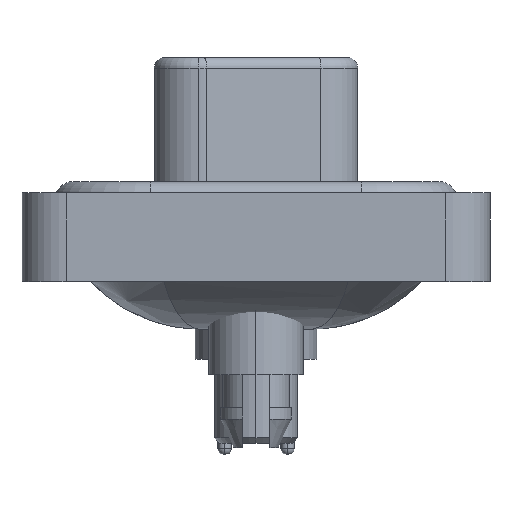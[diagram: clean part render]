
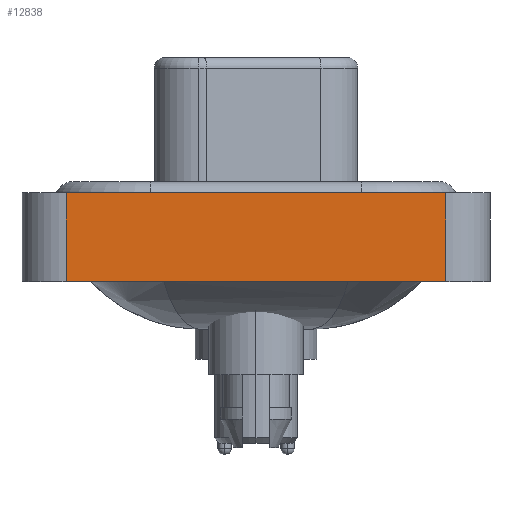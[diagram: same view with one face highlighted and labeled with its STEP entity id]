
A CAD part, left-side view. The second image highlights one B-rep face of the part: STEP entity #12838.
In plain terms, the highlighted planar face has unit normal (-1, 0, 0).
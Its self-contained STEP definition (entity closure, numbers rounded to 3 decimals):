
#242 = DIRECTION ( 'NONE',  ( 0., -1., 0. ) ) ;
#1107 = ORIENTED_EDGE ( 'NONE', *, *, #14644, .F. ) ;
#1788 = FACE_OUTER_BOUND ( 'NONE', #9167, .T. ) ;
#2970 = VERTEX_POINT ( 'NONE', #6866 ) ;
#3926 = VERTEX_POINT ( 'NONE', #19527 ) ;
#4065 = VECTOR ( 'NONE', #242, 1000. ) ;
#4536 = EDGE_CURVE ( 'NONE', #9618, #3926, #15496, .T. ) ;
#5072 = CARTESIAN_POINT ( 'NONE',  ( -7.3, -8.55, -3.6 ) ) ;
#5368 = LINE ( 'NONE', #8829, #6165 ) ;
#6165 = VECTOR ( 'NONE', #19513, 1000. ) ;
#6378 = LINE ( 'NONE', #14205, #4065 ) ;
#6866 = CARTESIAN_POINT ( 'NONE',  ( -7.3, -8.55, 0.4 ) ) ;
#8171 = CARTESIAN_POINT ( 'NONE',  ( -7.3, -8.55, -3.6 ) ) ;
#8829 = CARTESIAN_POINT ( 'NONE',  ( -7.3, -8.55, 0.4 ) ) ;
#9164 = VERTEX_POINT ( 'NONE', #8171 ) ;
#9167 = EDGE_LOOP ( 'NONE', ( #17342, #1107, #18517, #16993 ) ) ;
#9552 = DIRECTION ( 'NONE',  ( 0., 0., 1. ) ) ;
#9618 = VERTEX_POINT ( 'NONE', #12909 ) ;
#11034 = DIRECTION ( 'NONE',  ( -1., 0., 0. ) ) ;
#11043 = VECTOR ( 'NONE', #9552, 1000. ) ;
#12065 = EDGE_CURVE ( 'NONE', #9618, #9164, #6378, .T. ) ;
#12542 = CARTESIAN_POINT ( 'NONE',  ( -7.3, 8.55, -3.6 ) ) ;
#12838 = ADVANCED_FACE ( 'NONE', ( #1788 ), #14113, .T. ) ;
#12909 = CARTESIAN_POINT ( 'NONE',  ( -7.3, 8.55, -3.6 ) ) ;
#14076 = VECTOR ( 'NONE', #17118, 1000. ) ;
#14113 = PLANE ( 'NONE',  #17730 ) ;
#14205 = CARTESIAN_POINT ( 'NONE',  ( -7.3, -8.55, -3.6 ) ) ;
#14644 = EDGE_CURVE ( 'NONE', #3926, #2970, #5368, .T. ) ;
#15496 = LINE ( 'NONE', #12542, #14076 ) ;
#16993 = ORIENTED_EDGE ( 'NONE', *, *, #12065, .T. ) ;
#17118 = DIRECTION ( 'NONE',  ( 0., 0., 1. ) ) ;
#17342 = ORIENTED_EDGE ( 'NONE', *, *, #17988, .T. ) ;
#17730 = AXIS2_PLACEMENT_3D ( 'NONE', #19190, #11034, #18783 ) ;
#17988 = EDGE_CURVE ( 'NONE', #9164, #2970, #18800, .T. ) ;
#18517 = ORIENTED_EDGE ( 'NONE', *, *, #4536, .F. ) ;
#18783 = DIRECTION ( 'NONE',  ( 0., 0., 1. ) ) ;
#18800 = LINE ( 'NONE', #5072, #11043 ) ;
#19190 = CARTESIAN_POINT ( 'NONE',  ( -7.3, -8.55, -3.6 ) ) ;
#19513 = DIRECTION ( 'NONE',  ( 0., -1., 0. ) ) ;
#19527 = CARTESIAN_POINT ( 'NONE',  ( -7.3, 8.55, 0.4 ) ) ;
